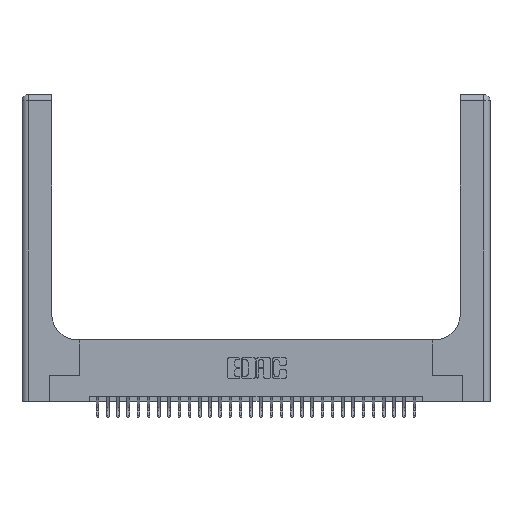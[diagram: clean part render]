
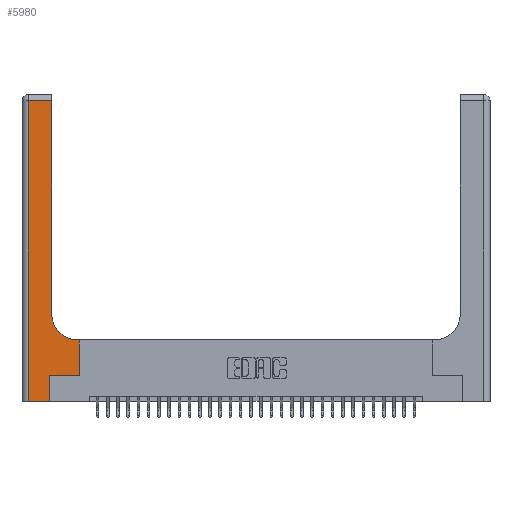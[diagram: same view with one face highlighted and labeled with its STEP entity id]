
A CAD part, top view. The second image highlights one B-rep face of the part: STEP entity #5980.
In plain terms, the highlighted planar face has unit normal (0, 0, 1).
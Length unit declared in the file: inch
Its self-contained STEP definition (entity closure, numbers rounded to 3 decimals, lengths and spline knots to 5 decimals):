
#546 = CARTESIAN_POINT ( 'NONE',  ( 0.2915, 3., 0.37 ) ) ;
#1004 = DIRECTION ( 'NONE',  ( 1., 0., 0. ) ) ;
#1369 = VECTOR ( 'NONE', #1004, 39.37008 ) ;
#2082 = VERTEX_POINT ( 'NONE', #13109 ) ;
#2291 = CARTESIAN_POINT ( 'NONE',  ( 0.269, 0.25, 0.37 ) ) ;
#2730 = EDGE_CURVE ( 'NONE', #4089, #29172, #29920, .T. ) ;
#3114 = CARTESIAN_POINT ( 'NONE',  ( 0.5585, 0.6, 0.37 ) ) ;
#3417 = EDGE_LOOP ( 'NONE', ( #25032, #29577, #25471, #11566, #20159, #30468, #15463, #30170, #28646 ) ) ;
#4089 = VERTEX_POINT ( 'NONE', #19077 ) ;
#4775 = EDGE_CURVE ( 'NONE', #22883, #24713, #13282, .T. ) ;
#5159 = EDGE_CURVE ( 'NONE', #2082, #17902, #19786, .T. ) ;
#5167 = LINE ( 'NONE', #27107, #12536 ) ;
#5411 = DIRECTION ( 'NONE',  ( -1., 0., 0. ) ) ;
#5980 = ADVANCED_FACE ( 'NONE', ( #18559 ), #27527, .F. ) ;
#8138 = LINE ( 'NONE', #12906, #17757 ) ;
#8223 = CARTESIAN_POINT ( 'NONE',  ( 0.2915, 0.85, 0.37 ) ) ;
#8231 = CARTESIAN_POINT ( 'NONE',  ( 0., 3., 0.37 ) ) ;
#8563 = EDGE_CURVE ( 'NONE', #29750, #2082, #13803, .T. ) ;
#10979 = CARTESIAN_POINT ( 'NONE',  ( 0.2915, 0.6, 0.37 ) ) ;
#11566 = ORIENTED_EDGE ( 'NONE', *, *, #8563, .T. ) ;
#12536 = VECTOR ( 'NONE', #14737, 39.37008 ) ;
#12906 = CARTESIAN_POINT ( 'NONE',  ( 0.5585, 0.25, 0.37 ) ) ;
#13109 = CARTESIAN_POINT ( 'NONE',  ( 0.269, 0., 0.37 ) ) ;
#13111 = LINE ( 'NONE', #10979, #15785 ) ;
#13282 = CIRCLE ( 'NONE', #20258, 0.25 ) ;
#13803 = LINE ( 'NONE', #23208, #1369 ) ;
#14006 = LINE ( 'NONE', #546, #24693 ) ;
#14737 = DIRECTION ( 'NONE',  ( 0., -1., 0. ) ) ;
#14766 = DIRECTION ( 'NONE',  ( 1., 0., 0. ) ) ;
#15113 = EDGE_CURVE ( 'NONE', #17902, #18203, #17532, .T. ) ;
#15379 = CARTESIAN_POINT ( 'NONE',  ( 0., 2.94, 0.37 ) ) ;
#15463 = ORIENTED_EDGE ( 'NONE', *, *, #18121, .T. ) ;
#15668 = DIRECTION ( 'NONE',  ( 0., 0., -1. ) ) ;
#15785 = VECTOR ( 'NONE', #22855, 39.37008 ) ;
#15959 = EDGE_CURVE ( 'NONE', #29172, #29750, #5167, .T. ) ;
#16070 = VERTEX_POINT ( 'NONE', #3114 ) ;
#17532 = LINE ( 'NONE', #23564, #29784 ) ;
#17757 = VECTOR ( 'NONE', #20608, 39.37008 ) ;
#17902 = VERTEX_POINT ( 'NONE', #2291 ) ;
#18121 = EDGE_CURVE ( 'NONE', #18203, #16070, #8138, .T. ) ;
#18203 = VERTEX_POINT ( 'NONE', #22852 ) ;
#18559 = FACE_OUTER_BOUND ( 'NONE', #3417, .T. ) ;
#18949 = CARTESIAN_POINT ( 'NONE',  ( 0.06, 2.94, 0.37 ) ) ;
#19077 = CARTESIAN_POINT ( 'NONE',  ( 0.2915, 2.94, 0.37 ) ) ;
#19786 = LINE ( 'NONE', #21323, #25487 ) ;
#20159 = ORIENTED_EDGE ( 'NONE', *, *, #5159, .T. ) ;
#20258 = AXIS2_PLACEMENT_3D ( 'NONE', #20835, #25155, #14766 ) ;
#20608 = DIRECTION ( 'NONE',  ( 0., 1., 0. ) ) ;
#20835 = CARTESIAN_POINT ( 'NONE',  ( 0.5415, 0.85, 0.37 ) ) ;
#20935 = CARTESIAN_POINT ( 'NONE',  ( 0.06, 0., 0.37 ) ) ;
#21323 = CARTESIAN_POINT ( 'NONE',  ( 0.269, 0., 0.37 ) ) ;
#21799 = EDGE_CURVE ( 'NONE', #24713, #4089, #14006, .T. ) ;
#22852 = CARTESIAN_POINT ( 'NONE',  ( 0.5585, 0.25, 0.37 ) ) ;
#22855 = DIRECTION ( 'NONE',  ( -1., 0., 0. ) ) ;
#22883 = VERTEX_POINT ( 'NONE', #29532 ) ;
#23208 = CARTESIAN_POINT ( 'NONE',  ( 0., 0., 0.37 ) ) ;
#23564 = CARTESIAN_POINT ( 'NONE',  ( 0.269, 0.25, 0.37 ) ) ;
#24308 = EDGE_CURVE ( 'NONE', #16070, #22883, #13111, .T. ) ;
#24693 = VECTOR ( 'NONE', #27768, 39.37008 ) ;
#24713 = VERTEX_POINT ( 'NONE', #8223 ) ;
#24773 = DIRECTION ( 'NONE',  ( -1., 0., 0. ) ) ;
#25032 = ORIENTED_EDGE ( 'NONE', *, *, #21799, .T. ) ;
#25155 = DIRECTION ( 'NONE',  ( 0., 0., -1. ) ) ;
#25337 = VECTOR ( 'NONE', #24773, 39.37008 ) ;
#25471 = ORIENTED_EDGE ( 'NONE', *, *, #15959, .T. ) ;
#25487 = VECTOR ( 'NONE', #29249, 39.37008 ) ;
#27107 = CARTESIAN_POINT ( 'NONE',  ( 0.06, 3., 0.37 ) ) ;
#27205 = AXIS2_PLACEMENT_3D ( 'NONE', #8231, #15668, #5411 ) ;
#27527 = PLANE ( 'NONE',  #27205 ) ;
#27768 = DIRECTION ( 'NONE',  ( 0., 1., 0. ) ) ;
#28646 = ORIENTED_EDGE ( 'NONE', *, *, #4775, .T. ) ;
#29172 = VERTEX_POINT ( 'NONE', #18949 ) ;
#29249 = DIRECTION ( 'NONE',  ( 0., 1., 0. ) ) ;
#29532 = CARTESIAN_POINT ( 'NONE',  ( 0.5415, 0.6, 0.37 ) ) ;
#29577 = ORIENTED_EDGE ( 'NONE', *, *, #2730, .T. ) ;
#29750 = VERTEX_POINT ( 'NONE', #20935 ) ;
#29784 = VECTOR ( 'NONE', #30951, 39.37008 ) ;
#29920 = LINE ( 'NONE', #15379, #25337 ) ;
#30170 = ORIENTED_EDGE ( 'NONE', *, *, #24308, .T. ) ;
#30468 = ORIENTED_EDGE ( 'NONE', *, *, #15113, .T. ) ;
#30951 = DIRECTION ( 'NONE',  ( 1., 0., 0. ) ) ;
